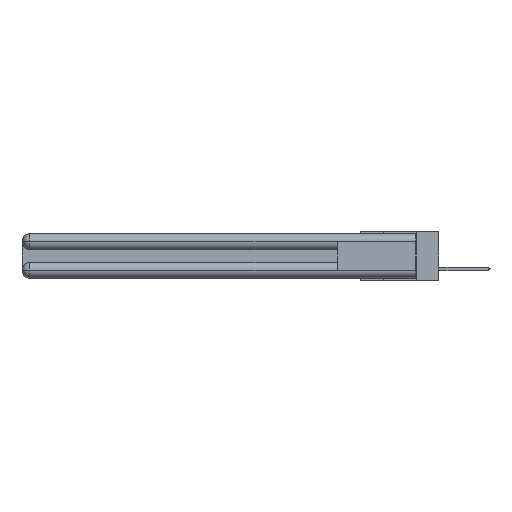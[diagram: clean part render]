
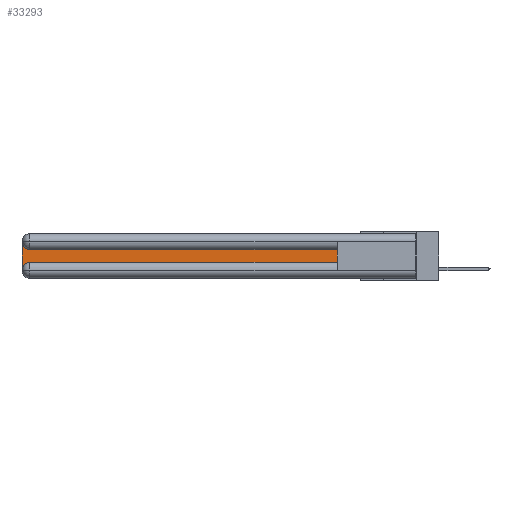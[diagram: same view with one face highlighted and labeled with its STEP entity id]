
A CAD part, left-side view. The second image highlights one B-rep face of the part: STEP entity #33293.
In plain terms, the highlighted planar face has unit normal (-1, 0, 0).
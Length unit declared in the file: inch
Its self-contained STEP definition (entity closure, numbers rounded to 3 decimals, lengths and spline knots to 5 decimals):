
#50 = ORIENTED_EDGE ( 'NONE', *, *, #9523, .T. ) ;
#2657 = DIRECTION ( 'NONE',  ( 0., 0., -1. ) ) ;
#4128 = AXIS2_PLACEMENT_3D ( 'NONE', #26079, #10339, #10456 ) ;
#4329 = LINE ( 'NONE', #7321, #23582 ) ;
#4451 = EDGE_CURVE ( 'NONE', #16753, #33438, #13345, .T. ) ;
#4565 = VERTEX_POINT ( 'NONE', #22277 ) ;
#4849 = EDGE_LOOP ( 'NONE', ( #15587, #12337, #18637, #22558, #50, #15629 ) ) ;
#5576 = DIRECTION ( 'NONE',  ( 1., 0., 0. ) ) ;
#6407 = CARTESIAN_POINT ( 'NONE',  ( 0.075, 0.6, -0.1225 ) ) ;
#7321 = CARTESIAN_POINT ( 'NONE',  ( 0.075, 0.6, -0.2175 ) ) ;
#9523 = EDGE_CURVE ( 'NONE', #4565, #16753, #4329, .T. ) ;
#10339 = DIRECTION ( 'NONE',  ( 1., 0., 0. ) ) ;
#10377 = VERTEX_POINT ( 'NONE', #30189 ) ;
#10456 = DIRECTION ( 'NONE',  ( 0., 0., -1. ) ) ;
#10547 = CARTESIAN_POINT ( 'NONE',  ( 0.075, 0.6, -0.2175 ) ) ;
#11403 = DIRECTION ( 'NONE',  ( 0., 1., 0. ) ) ;
#12337 = ORIENTED_EDGE ( 'NONE', *, *, #19105, .T. ) ;
#13345 = LINE ( 'NONE', #21599, #20336 ) ;
#13749 = LINE ( 'NONE', #32008, #26048 ) ;
#13855 = CARTESIAN_POINT ( 'NONE',  ( 0.075, 2.94, -0.1225 ) ) ;
#13906 = DIRECTION ( 'NONE',  ( 0., 0., -1. ) ) ;
#14881 = DIRECTION ( 'NONE',  ( 0., -1., 0. ) ) ;
#15587 = ORIENTED_EDGE ( 'NONE', *, *, #16270, .T. ) ;
#15629 = ORIENTED_EDGE ( 'NONE', *, *, #4451, .T. ) ;
#16270 = EDGE_CURVE ( 'NONE', #33438, #33806, #18177, .T. ) ;
#16332 = AXIS2_PLACEMENT_3D ( 'NONE', #34031, #23168, #2657 ) ;
#16753 = VERTEX_POINT ( 'NONE', #10547 ) ;
#17640 = VERTEX_POINT ( 'NONE', #31930 ) ;
#18177 = LINE ( 'NONE', #6407, #27307 ) ;
#18448 = CARTESIAN_POINT ( 'NONE',  ( 0.075, 0.6, -0.1225 ) ) ;
#18637 = ORIENTED_EDGE ( 'NONE', *, *, #30863, .T. ) ;
#19105 = EDGE_CURVE ( 'NONE', #33806, #17640, #22168, .T. ) ;
#19776 = EDGE_CURVE ( 'NONE', #10377, #4565, #21230, .T. ) ;
#20336 = VECTOR ( 'NONE', #24367, 39.37008 ) ;
#21230 = CIRCLE ( 'NONE', #4128, 0.06 ) ;
#21599 = CARTESIAN_POINT ( 'NONE',  ( 0.075, 0.6, -0.2175 ) ) ;
#22168 = CIRCLE ( 'NONE', #23650, 0.06 ) ;
#22277 = CARTESIAN_POINT ( 'NONE',  ( 0.075, 2.94, -0.2175 ) ) ;
#22558 = ORIENTED_EDGE ( 'NONE', *, *, #19776, .T. ) ;
#23168 = DIRECTION ( 'NONE',  ( 1., 0., 0. ) ) ;
#23582 = VECTOR ( 'NONE', #14881, 39.37008 ) ;
#23650 = AXIS2_PLACEMENT_3D ( 'NONE', #29416, #5576, #27014 ) ;
#24367 = DIRECTION ( 'NONE',  ( 0., 0., 1. ) ) ;
#26048 = VECTOR ( 'NONE', #13906, 39.37008 ) ;
#26079 = CARTESIAN_POINT ( 'NONE',  ( 0.075, 2.94, -0.2775 ) ) ;
#26474 = FACE_OUTER_BOUND ( 'NONE', #4849, .T. ) ;
#27014 = DIRECTION ( 'NONE',  ( 0., 0., -1. ) ) ;
#27307 = VECTOR ( 'NONE', #11403, 39.37008 ) ;
#29416 = CARTESIAN_POINT ( 'NONE',  ( 0.075, 2.94, -0.0625 ) ) ;
#30189 = CARTESIAN_POINT ( 'NONE',  ( 0.075, 3., -0.2775 ) ) ;
#30863 = EDGE_CURVE ( 'NONE', #17640, #10377, #13749, .T. ) ;
#31283 = PLANE ( 'NONE',  #16332 ) ;
#31930 = CARTESIAN_POINT ( 'NONE',  ( 0.075, 3., -0.0625 ) ) ;
#32008 = CARTESIAN_POINT ( 'NONE',  ( 0.075, 3., -0.2175 ) ) ;
#33293 = ADVANCED_FACE ( 'NONE', ( #26474 ), #31283, .F. ) ;
#33438 = VERTEX_POINT ( 'NONE', #18448 ) ;
#33806 = VERTEX_POINT ( 'NONE', #13855 ) ;
#34031 = CARTESIAN_POINT ( 'NONE',  ( 0.075, 3., -0.1225 ) ) ;
